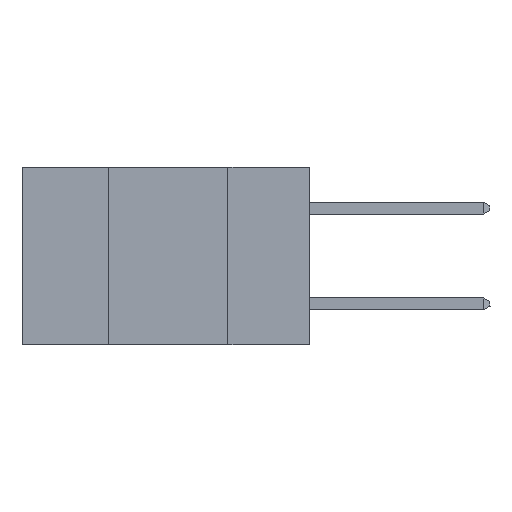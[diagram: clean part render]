
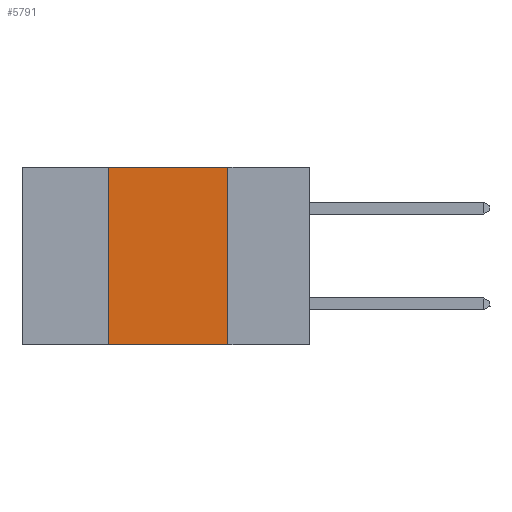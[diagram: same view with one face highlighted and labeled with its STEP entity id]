
A CAD part, left-side view. The second image highlights one B-rep face of the part: STEP entity #5791.
In plain terms, the highlighted planar face has unit normal (-1, 0, 0).
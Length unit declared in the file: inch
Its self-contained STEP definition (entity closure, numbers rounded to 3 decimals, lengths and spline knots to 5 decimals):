
#195 = AXIS2_PLACEMENT_3D ( 'NONE', #4417, #9963, #2005 ) ;
#357 = VERTEX_POINT ( 'NONE', #7731 ) ;
#423 = VECTOR ( 'NONE', #8824, 39.37008 ) ;
#452 = LINE ( 'NONE', #2203, #2069 ) ;
#795 = ORIENTED_EDGE ( 'NONE', *, *, #918, .F. ) ;
#800 = CARTESIAN_POINT ( 'NONE',  ( 0., 0.42, -0.37 ) ) ;
#918 = EDGE_CURVE ( 'NONE', #5453, #6542, #9846, .T. ) ;
#1224 = DIRECTION ( 'NONE',  ( 0., -1., 0. ) ) ;
#1926 = CARTESIAN_POINT ( 'NONE',  ( 0., 0.42, 0. ) ) ;
#2005 = DIRECTION ( 'NONE',  ( 0., 0., -1. ) ) ;
#2069 = VECTOR ( 'NONE', #7653, 39.37008 ) ;
#2203 = CARTESIAN_POINT ( 'NONE',  ( 0., 0.6, 0. ) ) ;
#2250 = EDGE_LOOP ( 'NONE', ( #7833, #10247, #795, #5408 ) ) ;
#2556 = VECTOR ( 'NONE', #1224, 39.37008 ) ;
#3438 = VERTEX_POINT ( 'NONE', #4182 ) ;
#4182 = CARTESIAN_POINT ( 'NONE',  ( 0., 0.17, 0. ) ) ;
#4404 = LINE ( 'NONE', #7612, #2556 ) ;
#4417 = CARTESIAN_POINT ( 'NONE',  ( 0., 0.6, 0. ) ) ;
#5408 = ORIENTED_EDGE ( 'NONE', *, *, #7215, .T. ) ;
#5453 = VERTEX_POINT ( 'NONE', #800 ) ;
#5791 = ADVANCED_FACE ( 'NONE', ( #8017 ), #6079, .F. ) ;
#6022 = CARTESIAN_POINT ( 'NONE',  ( 0., 0.17, 0. ) ) ;
#6079 = PLANE ( 'NONE',  #195 ) ;
#6237 = DIRECTION ( 'NONE',  ( 0., 0., -1. ) ) ;
#6272 = EDGE_CURVE ( 'NONE', #6542, #3438, #452, .T. ) ;
#6542 = VERTEX_POINT ( 'NONE', #1926 ) ;
#6716 = EDGE_CURVE ( 'NONE', #3438, #357, #9724, .T. ) ;
#7215 = EDGE_CURVE ( 'NONE', #5453, #357, #4404, .T. ) ;
#7495 = VECTOR ( 'NONE', #6237, 39.37008 ) ;
#7612 = CARTESIAN_POINT ( 'NONE',  ( 0., 0.6, -0.37 ) ) ;
#7653 = DIRECTION ( 'NONE',  ( 0., -1., 0. ) ) ;
#7731 = CARTESIAN_POINT ( 'NONE',  ( 0., 0.17, -0.37 ) ) ;
#7833 = ORIENTED_EDGE ( 'NONE', *, *, #6716, .F. ) ;
#8017 = FACE_OUTER_BOUND ( 'NONE', #2250, .T. ) ;
#8019 = CARTESIAN_POINT ( 'NONE',  ( 0., 0.42, 0. ) ) ;
#8824 = DIRECTION ( 'NONE',  ( 0., 0., 1. ) ) ;
#9724 = LINE ( 'NONE', #6022, #7495 ) ;
#9846 = LINE ( 'NONE', #8019, #423 ) ;
#9963 = DIRECTION ( 'NONE',  ( 1., 0., 0. ) ) ;
#10247 = ORIENTED_EDGE ( 'NONE', *, *, #6272, .F. ) ;
